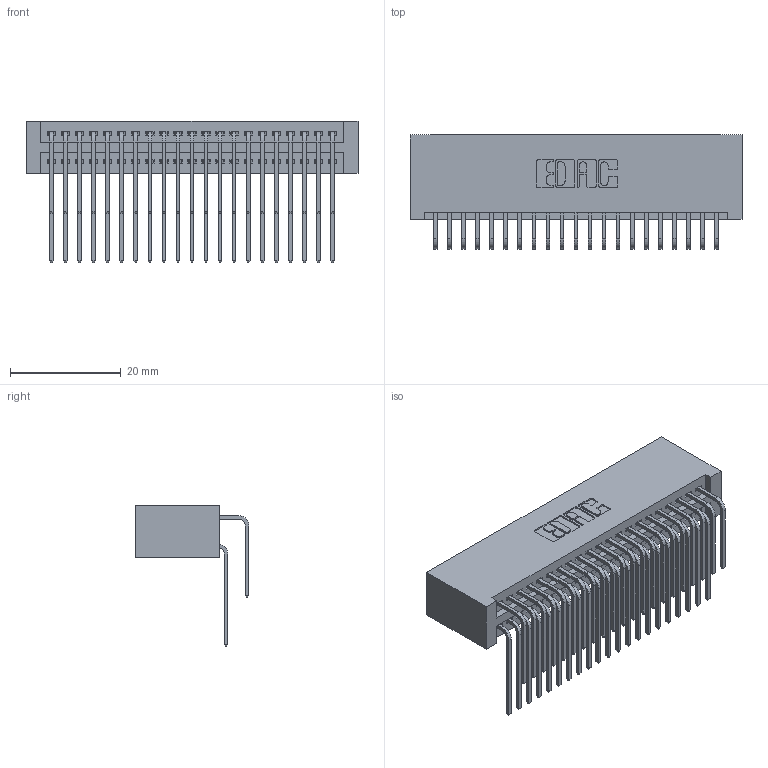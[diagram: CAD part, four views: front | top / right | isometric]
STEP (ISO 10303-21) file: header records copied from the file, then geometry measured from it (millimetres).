
FILE_DESCRIPTION (( 'STEP AP203' ), '1' );
FILE_NAME ('345-042-559-201.STEP', '2018-09-08T00:53:19', ( '' ), ( '' ), 'SwSTEP 2.0', 'SolidWorks 2016', '' );
FILE_SCHEMA (( 'CONFIG_CONTROL_DESIGN' ));
Length unit declared in the file: inch
Products named in the file (4): 345 Part_No Mounting Lugs; 345-292-001_558 559 Tail - 1; 345-292-001_559 Tail - 2; 345-042-559-201
Assembly tree (43 placements, depth 2):
  345-042-559-201
    345 Part_No Mounting Lugs
    345-292-001_558 559 Tail - 1  x21
    345-292-001_559 Tail - 2  x21
Bounding box: 59.94 x 20.56 x 25.53 mm (x, y, z)
Volume: 6486.3 mm3; surface area: 10623.7 mm2
Topology: 43 solids, 43 shells, 2302 faces, 6827 edges, 4494 vertices
Faces by surface type: plane 1546, cylinder 756
Entity records: 20679 total; most frequent: CARTESIAN_POINT 3531, ORIENTED_EDGE 3414, DIRECTION 3107, EDGE_CURVE 1707, VECTOR 1459, LINE 1459, VERTEX_POINT 1134, AXIS2_PLACEMENT_3D 824
